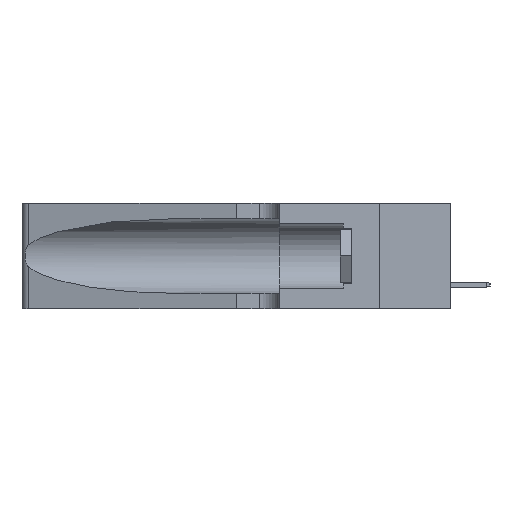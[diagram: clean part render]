
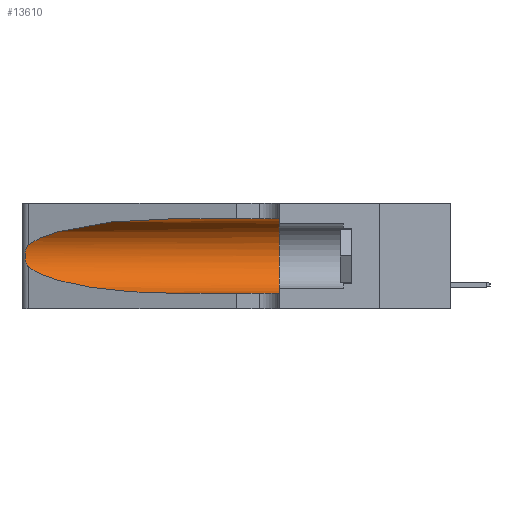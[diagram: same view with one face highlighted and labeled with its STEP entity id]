
A CAD part, left-side view. The second image highlights one B-rep face of the part: STEP entity #13610.
In plain terms, the highlighted cylindrical face has radius 3.308 mm (diameter 6.617 mm), a partial arc.
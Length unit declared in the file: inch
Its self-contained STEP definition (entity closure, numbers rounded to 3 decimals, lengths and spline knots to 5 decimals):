
#92 = EDGE_LOOP ( 'NONE', ( #16224, #653, #14383, #7058, #14354, #11344 ) ) ;
#223 = DIRECTION ( 'NONE',  ( 0., 0., 1. ) ) ;
#412 = CARTESIAN_POINT ( 'NONE',  ( 0.25856, 1.23593, 0.16098 ) ) ;
#653 = ORIENTED_EDGE ( 'NONE', *, *, #1850, .T. ) ;
#677 = CARTESIAN_POINT ( 'NONE',  ( 0.26018, 1.23835, 0.19895 ) ) ;
#1497 = DIRECTION ( 'NONE',  ( 0., 0., -1. ) ) ;
#1758 = CARTESIAN_POINT ( 'NONE',  ( 0.25789, 1.23486, 0.15765 ) ) ;
#1850 = EDGE_CURVE ( 'NONE', #11844, #13843, #13011, .T. ) ;
#1903 = CARTESIAN_POINT ( 'NONE',  ( 0.1305, 1.61858, 0.05475 ) ) ;
#1942 = CARTESIAN_POINT ( 'NONE',  ( 0.25854, 1.2359, 0.20912 ) ) ;
#1996 = CARTESIAN_POINT ( 'NONE',  ( 0.25487, 1.22718, 0.22369 ) ) ;
#2088 = CARTESIAN_POINT ( 'NONE',  ( 0.2373, 1.15595, 0.28018 ) ) ;
#2345 = CIRCLE ( 'NONE', #9840, 0.13025 ) ;
#2495 = EDGE_CURVE ( 'NONE', #10857, #12264, #12446, .T. ) ;
#2617 = EDGE_CURVE ( 'NONE', #13292, #7937, #4470, .T. ) ;
#3077 = CARTESIAN_POINT ( 'NONE',  ( 0.1305, 0.72297, 0.31525 ) ) ;
#4337 = CARTESIAN_POINT ( 'NONE',  ( 0.1305, 1.61858, 0.185 ) ) ;
#4470 = LINE ( 'NONE', #1903, #17394 ) ;
#4691 = CARTESIAN_POINT ( 'NONE',  ( 0.25555, 1.22994, 0.2215 ) ) ;
#4778 = CARTESIAN_POINT ( 'NONE',  ( 0.26017, 1.23833, 0.17102 ) ) ;
#5908 = EDGE_CURVE ( 'NONE', #13843, #13292, #17207, .T. ) ;
#5981 = DIRECTION ( 'NONE',  ( 0., -1., 0. ) ) ;
#6326 = CARTESIAN_POINT ( 'NONE',  ( 0.1305, 0.72297, 0.05475 ) ) ;
#6957 = CARTESIAN_POINT ( 'NONE',  ( 0.1305, 0.35, 0.185 ) ) ;
#6958 =( BOUNDED_CURVE ( )  B_SPLINE_CURVE ( 3, ( #17276, #14328, #2088, #1996 ),
 .UNSPECIFIED., .F., .F. ) 
 B_SPLINE_CURVE_WITH_KNOTS ( ( 4, 4 ),
 ( 1.5708, 2.84003 ),
 .UNSPECIFIED. ) 
 CURVE ( )  GEOMETRIC_REPRESENTATION_ITEM ( )  RATIONAL_B_SPLINE_CURVE ( ( 1., 0.87, 0.87, 1. ) ) 
 REPRESENTATION_ITEM ( '' )  );
#7058 = ORIENTED_EDGE ( 'NONE', *, *, #2617, .T. ) ;
#7279 = CARTESIAN_POINT ( 'NONE',  ( 0.18966, 0.96281, 0.05475 ) ) ;
#7324 = CARTESIAN_POINT ( 'NONE',  ( 0.26075, 1.23896, 0.19203 ) ) ;
#7416 = CARTESIAN_POINT ( 'NONE',  ( 0.25787, 1.23484, 0.2124 ) ) ;
#7894 = CARTESIAN_POINT ( 'NONE',  ( 0.2373, 1.15595, 0.08982 ) ) ;
#7937 = VERTEX_POINT ( 'NONE', #10472 ) ;
#8179 = CARTESIAN_POINT ( 'NONE',  ( 0.25487, 1.22718, 0.22369 ) ) ;
#8285 = CARTESIAN_POINT ( 'NONE',  ( 0.1305, 1.61858, 0.31525 ) ) ;
#8589 = CARTESIAN_POINT ( 'NONE',  ( 0.25487, 1.22718, 0.22369 ) ) ;
#8936 = CARTESIAN_POINT ( 'NONE',  ( 0.25639, 1.23186, 0.15144 ) ) ;
#9641 = VECTOR ( 'NONE', #11177, 39.37008 ) ;
#9706 = EDGE_CURVE ( 'NONE', #10857, #11844, #6958, .T. ) ;
#9840 = AXIS2_PLACEMENT_3D ( 'NONE', #6957, #11480, #223 ) ;
#9877 = DIRECTION ( 'NONE',  ( 0., -1., 0. ) ) ;
#10392 = CARTESIAN_POINT ( 'NONE',  ( 0.25487, 1.22718, 0.14631 ) ) ;
#10472 = CARTESIAN_POINT ( 'NONE',  ( 0.1305, 0.35, 0.05475 ) ) ;
#10857 = VERTEX_POINT ( 'NONE', #3077 ) ;
#11177 = DIRECTION ( 'NONE',  ( 0., -1., 0. ) ) ;
#11344 = ORIENTED_EDGE ( 'NONE', *, *, #2495, .F. ) ;
#11480 = DIRECTION ( 'NONE',  ( 0., 1., 0. ) ) ;
#11844 = VERTEX_POINT ( 'NONE', #8179 ) ;
#12264 = VERTEX_POINT ( 'NONE', #12742 ) ;
#12446 = LINE ( 'NONE', #8285, #9641 ) ;
#12742 = CARTESIAN_POINT ( 'NONE',  ( 0.1305, 0.35, 0.31525 ) ) ;
#12858 = CARTESIAN_POINT ( 'NONE',  ( 0.26075, 1.23896, 0.178 ) ) ;
#13011 = B_SPLINE_CURVE_WITH_KNOTS ( 'NONE', 3,
 ( #8589, #4691, #15514, #7416, #1942, #677, #7324, #12858, #4778, #412, #1758, #8936, #15777, #14279 ),
 .UNSPECIFIED., .F., .F.,
 ( 4, 2, 2, 2, 2, 2, 4 ),
 ( 0., 0.00027, 0.00053, 0.00107, 0.0016, 0.00187, 0.00214 ),
 .UNSPECIFIED. ) ;
#13292 = VERTEX_POINT ( 'NONE', #17240 ) ;
#13610 = ADVANCED_FACE ( 'NONE', ( #15168 ), #16421, .F. ) ;
#13843 = VERTEX_POINT ( 'NONE', #10392 ) ;
#14100 = AXIS2_PLACEMENT_3D ( 'NONE', #4337, #9877, #1497 ) ;
#14279 = CARTESIAN_POINT ( 'NONE',  ( 0.25487, 1.22718, 0.14631 ) ) ;
#14328 = CARTESIAN_POINT ( 'NONE',  ( 0.18966, 0.96281, 0.31525 ) ) ;
#14354 = ORIENTED_EDGE ( 'NONE', *, *, #17227, .F. ) ;
#14383 = ORIENTED_EDGE ( 'NONE', *, *, #5908, .T. ) ;
#15168 = FACE_OUTER_BOUND ( 'NONE', #92, .T. ) ;
#15514 = CARTESIAN_POINT ( 'NONE',  ( 0.25639, 1.23184, 0.21858 ) ) ;
#15777 = CARTESIAN_POINT ( 'NONE',  ( 0.25555, 1.22993, 0.14849 ) ) ;
#16157 = CARTESIAN_POINT ( 'NONE',  ( 0.25487, 1.22718, 0.14631 ) ) ;
#16224 = ORIENTED_EDGE ( 'NONE', *, *, #9706, .T. ) ;
#16421 = CYLINDRICAL_SURFACE ( 'NONE', #14100, 0.13025 ) ;
#17207 =( BOUNDED_CURVE ( )  B_SPLINE_CURVE ( 3, ( #16157, #7894, #7279, #6326 ),
 .UNSPECIFIED., .F., .F. ) 
 B_SPLINE_CURVE_WITH_KNOTS ( ( 4, 4 ),
 ( 3.44316, 4.71239 ),
 .UNSPECIFIED. ) 
 CURVE ( )  GEOMETRIC_REPRESENTATION_ITEM ( )  RATIONAL_B_SPLINE_CURVE ( ( 1., 0.87, 0.87, 1. ) ) 
 REPRESENTATION_ITEM ( '' )  );
#17227 = EDGE_CURVE ( 'NONE', #12264, #7937, #2345, .T. ) ;
#17240 = CARTESIAN_POINT ( 'NONE',  ( 0.1305, 0.72297, 0.05475 ) ) ;
#17276 = CARTESIAN_POINT ( 'NONE',  ( 0.1305, 0.72297, 0.31525 ) ) ;
#17394 = VECTOR ( 'NONE', #5981, 39.37008 ) ;
